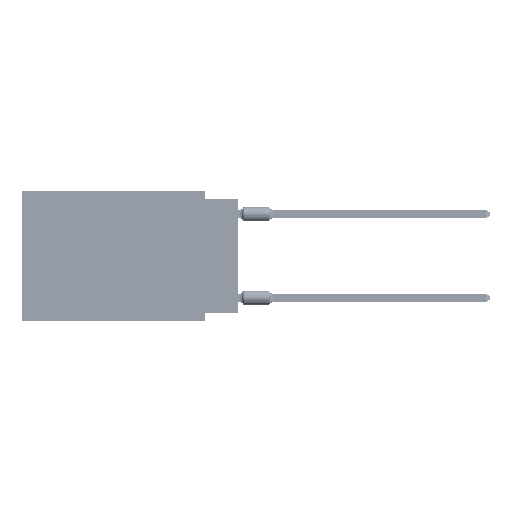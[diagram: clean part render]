
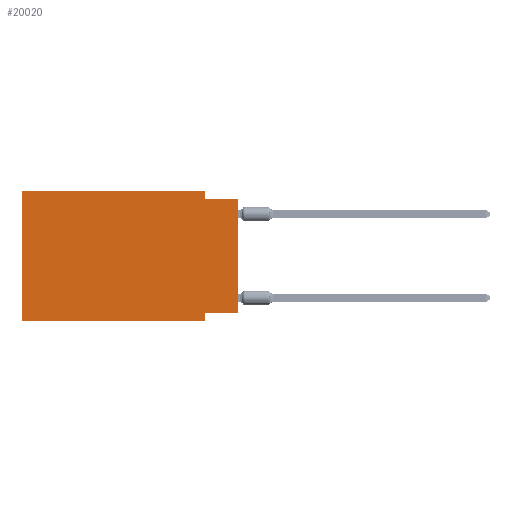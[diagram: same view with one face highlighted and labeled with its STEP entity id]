
A CAD part, left-side view. The second image highlights one B-rep face of the part: STEP entity #20020.
In plain terms, the highlighted planar face has unit normal (-1, 0, 0).
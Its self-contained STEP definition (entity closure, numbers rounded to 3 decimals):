
#1427 = DIRECTION ( 'NONE',  ( 0., 0., -1. ) ) ;
#2143 = CARTESIAN_POINT ( 'NONE',  ( 0., 16.383, 0. ) ) ;
#3463 = EDGE_CURVE ( 'NONE', #54849, #34281, #20173, .T. ) ;
#7606 = CARTESIAN_POINT ( 'NONE',  ( 0., 0., -0.635 ) ) ;
#8309 = VERTEX_POINT ( 'NONE', #20651 ) ;
#9445 = CARTESIAN_POINT ( 'NONE',  ( 0., 0., -0.635 ) ) ;
#9803 = LINE ( 'NONE', #9445, #15152 ) ;
#10821 = AXIS2_PLACEMENT_3D ( 'NONE', #66627, #33864, #1427 ) ;
#11134 = VERTEX_POINT ( 'NONE', #14180 ) ;
#11552 = VECTOR ( 'NONE', #14156, 1000. ) ;
#11761 = LINE ( 'NONE', #27789, #37012 ) ;
#14156 = DIRECTION ( 'NONE',  ( 0., 0., -1. ) ) ;
#14180 = CARTESIAN_POINT ( 'NONE',  ( 0., 2.54, 0. ) ) ;
#14743 = VECTOR ( 'NONE', #54965, 1000. ) ;
#15152 = VECTOR ( 'NONE', #15506, 1000. ) ;
#15506 = DIRECTION ( 'NONE',  ( 0., -1., 0. ) ) ;
#17663 = LINE ( 'NONE', #60783, #48141 ) ;
#17873 = EDGE_CURVE ( 'NONE', #65134, #47649, #9803, .T. ) ;
#19283 = CARTESIAN_POINT ( 'NONE',  ( 0., 0., 0. ) ) ;
#20020 = ADVANCED_FACE ( 'NONE', ( #50229 ), #32781, .F. ) ;
#20061 = EDGE_CURVE ( 'NONE', #59236, #34281, #11761, .T. ) ;
#20173 = LINE ( 'NONE', #55943, #35761 ) ;
#20651 = CARTESIAN_POINT ( 'NONE',  ( 0., 16.383, 0. ) ) ;
#21238 = CARTESIAN_POINT ( 'NONE',  ( 0., 2.54, -9.906 ) ) ;
#21878 = VECTOR ( 'NONE', #62677, 1000. ) ;
#25391 = ORIENTED_EDGE ( 'NONE', *, *, #3463, .T. ) ;
#27789 = CARTESIAN_POINT ( 'NONE',  ( 0., 2.54, -9.906 ) ) ;
#28948 = LINE ( 'NONE', #50324, #14743 ) ;
#30522 = CARTESIAN_POINT ( 'NONE',  ( 0., 16.383, -9.906 ) ) ;
#31293 = CARTESIAN_POINT ( 'NONE',  ( 0., 2.54, -0.635 ) ) ;
#32781 = PLANE ( 'NONE',  #10821 ) ;
#33864 = DIRECTION ( 'NONE',  ( 1., 0., 0. ) ) ;
#34281 = VERTEX_POINT ( 'NONE', #21238 ) ;
#35761 = VECTOR ( 'NONE', #68626, 1000. ) ;
#35887 = VECTOR ( 'NONE', #58101, 1000. ) ;
#37012 = VECTOR ( 'NONE', #43455, 1000. ) ;
#37596 = ORIENTED_EDGE ( 'NONE', *, *, #52937, .F. ) ;
#37954 = EDGE_CURVE ( 'NONE', #54849, #8309, #28948, .T. ) ;
#40931 = LINE ( 'NONE', #2143, #21878 ) ;
#41363 = VERTEX_POINT ( 'NONE', #54087 ) ;
#42056 = LINE ( 'NONE', #19283, #35887 ) ;
#43455 = DIRECTION ( 'NONE',  ( 0., 0., -1. ) ) ;
#47649 = VERTEX_POINT ( 'NONE', #7606 ) ;
#48141 = VECTOR ( 'NONE', #65762, 1000. ) ;
#50229 = FACE_OUTER_BOUND ( 'NONE', #54233, .T. ) ;
#50324 = CARTESIAN_POINT ( 'NONE',  ( 0., 16.383, 0. ) ) ;
#52242 = ORIENTED_EDGE ( 'NONE', *, *, #55917, .F. ) ;
#52296 = ORIENTED_EDGE ( 'NONE', *, *, #17873, .F. ) ;
#52937 = EDGE_CURVE ( 'NONE', #8309, #11134, #40931, .T. ) ;
#54087 = CARTESIAN_POINT ( 'NONE',  ( 0., 0., -9.271 ) ) ;
#54233 = EDGE_LOOP ( 'NONE', ( #68529, #52296, #52242, #37596, #63075, #25391, #61895, #60374 ) ) ;
#54849 = VERTEX_POINT ( 'NONE', #30522 ) ;
#54965 = DIRECTION ( 'NONE',  ( 0., 0., 1. ) ) ;
#55917 = EDGE_CURVE ( 'NONE', #11134, #65134, #56915, .T. ) ;
#55943 = CARTESIAN_POINT ( 'NONE',  ( 0., 16.383, -9.906 ) ) ;
#56915 = LINE ( 'NONE', #62957, #11552 ) ;
#58101 = DIRECTION ( 'NONE',  ( 0., 0., 1. ) ) ;
#59162 = CARTESIAN_POINT ( 'NONE',  ( 0., 2.54, -9.271 ) ) ;
#59236 = VERTEX_POINT ( 'NONE', #59162 ) ;
#60374 = ORIENTED_EDGE ( 'NONE', *, *, #67126, .F. ) ;
#60783 = CARTESIAN_POINT ( 'NONE',  ( 0., 0., -9.271 ) ) ;
#61895 = ORIENTED_EDGE ( 'NONE', *, *, #20061, .F. ) ;
#62677 = DIRECTION ( 'NONE',  ( 0., -1., 0. ) ) ;
#62957 = CARTESIAN_POINT ( 'NONE',  ( 0., 2.54, 0. ) ) ;
#63075 = ORIENTED_EDGE ( 'NONE', *, *, #37954, .F. ) ;
#65134 = VERTEX_POINT ( 'NONE', #31293 ) ;
#65762 = DIRECTION ( 'NONE',  ( 0., 1., 0. ) ) ;
#66627 = CARTESIAN_POINT ( 'NONE',  ( 0., 16.383, 0. ) ) ;
#67126 = EDGE_CURVE ( 'NONE', #41363, #59236, #17663, .T. ) ;
#68529 = ORIENTED_EDGE ( 'NONE', *, *, #69730, .T. ) ;
#68626 = DIRECTION ( 'NONE',  ( 0., -1., 0. ) ) ;
#69730 = EDGE_CURVE ( 'NONE', #41363, #47649, #42056, .T. ) ;
